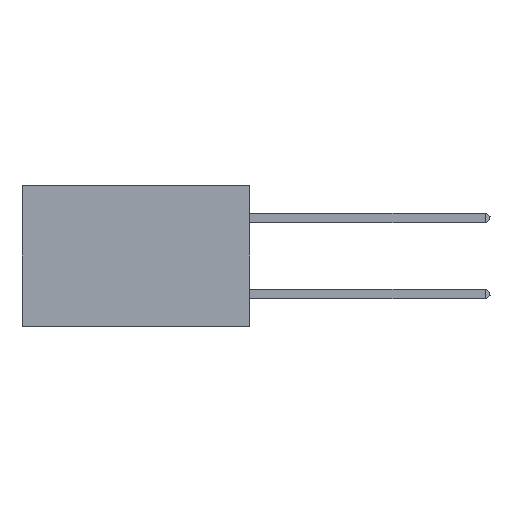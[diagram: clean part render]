
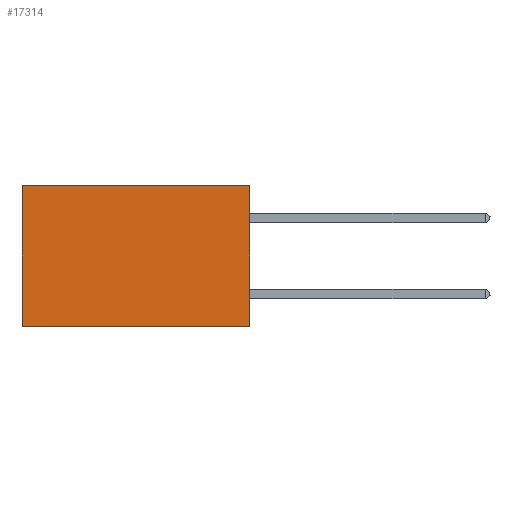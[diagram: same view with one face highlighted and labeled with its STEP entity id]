
A CAD part, left-side view. The second image highlights one B-rep face of the part: STEP entity #17314.
In plain terms, the highlighted planar face has unit normal (-1, 0, 0).
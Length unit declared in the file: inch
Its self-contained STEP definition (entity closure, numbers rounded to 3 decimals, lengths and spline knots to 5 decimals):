
#512 = ORIENTED_EDGE ( 'NONE', *, *, #24128, .T. ) ;
#520 = CARTESIAN_POINT ( 'NONE',  ( 0.2875, 0.6, -0.37 ) ) ;
#661 = LINE ( 'NONE', #11903, #31825 ) ;
#2874 = CARTESIAN_POINT ( 'NONE',  ( 0.2875, 0., -0.37 ) ) ;
#6204 = ORIENTED_EDGE ( 'NONE', *, *, #19017, .F. ) ;
#7116 = ORIENTED_EDGE ( 'NONE', *, *, #14604, .F. ) ;
#8112 = DIRECTION ( 'NONE',  ( 1., 0., 0. ) ) ;
#8738 = EDGE_CURVE ( 'NONE', #31269, #31493, #27068, .T. ) ;
#9159 = CARTESIAN_POINT ( 'NONE',  ( 0.2875, 0.6, 0. ) ) ;
#10168 = LINE ( 'NONE', #16136, #19291 ) ;
#10869 = VERTEX_POINT ( 'NONE', #16962 ) ;
#11903 = CARTESIAN_POINT ( 'NONE',  ( 0.2875, 0., 0. ) ) ;
#12233 = DIRECTION ( 'NONE',  ( 0., 1., 0. ) ) ;
#12972 = ORIENTED_EDGE ( 'NONE', *, *, #8738, .T. ) ;
#13691 = AXIS2_PLACEMENT_3D ( 'NONE', #20405, #8112, #19898 ) ;
#14604 = EDGE_CURVE ( 'NONE', #31269, #10869, #661, .T. ) ;
#16136 = CARTESIAN_POINT ( 'NONE',  ( 0.2875, 0.6, 0. ) ) ;
#16962 = CARTESIAN_POINT ( 'NONE',  ( 0.2875, 0., -0.37 ) ) ;
#17314 = ADVANCED_FACE ( 'NONE', ( #21043 ), #23220, .F. ) ;
#17445 = CARTESIAN_POINT ( 'NONE',  ( 0.2875, 0., 0. ) ) ;
#19017 = EDGE_CURVE ( 'NONE', #10869, #27509, #19243, .T. ) ;
#19243 = LINE ( 'NONE', #2874, #29844 ) ;
#19264 = VECTOR ( 'NONE', #12233, 39.37008 ) ;
#19291 = VECTOR ( 'NONE', #28057, 39.37008 ) ;
#19898 = DIRECTION ( 'NONE',  ( 0., 0., -1. ) ) ;
#20405 = CARTESIAN_POINT ( 'NONE',  ( 0.2875, 0., 0. ) ) ;
#21043 = FACE_OUTER_BOUND ( 'NONE', #22528, .T. ) ;
#22528 = EDGE_LOOP ( 'NONE', ( #512, #6204, #7116, #12972 ) ) ;
#23065 = DIRECTION ( 'NONE',  ( 0., 1., 0. ) ) ;
#23220 = PLANE ( 'NONE',  #13691 ) ;
#24128 = EDGE_CURVE ( 'NONE', #31493, #27509, #10168, .T. ) ;
#24286 = CARTESIAN_POINT ( 'NONE',  ( 0.2875, 0., 0. ) ) ;
#27068 = LINE ( 'NONE', #24286, #19264 ) ;
#27509 = VERTEX_POINT ( 'NONE', #520 ) ;
#28057 = DIRECTION ( 'NONE',  ( 0., 0., -1. ) ) ;
#29844 = VECTOR ( 'NONE', #23065, 39.37008 ) ;
#31269 = VERTEX_POINT ( 'NONE', #17445 ) ;
#31493 = VERTEX_POINT ( 'NONE', #9159 ) ;
#31825 = VECTOR ( 'NONE', #32666, 39.37008 ) ;
#32666 = DIRECTION ( 'NONE',  ( 0., 0., -1. ) ) ;
